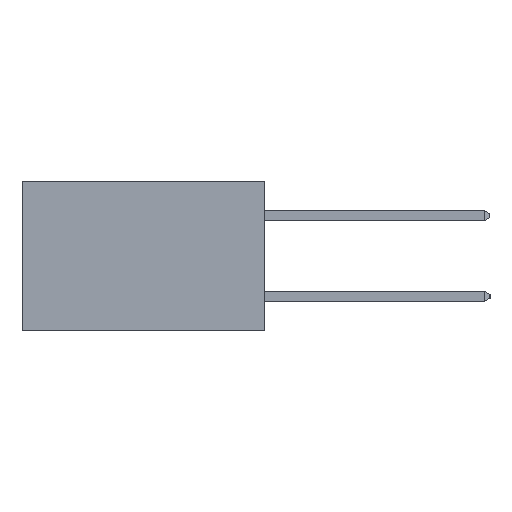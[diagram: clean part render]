
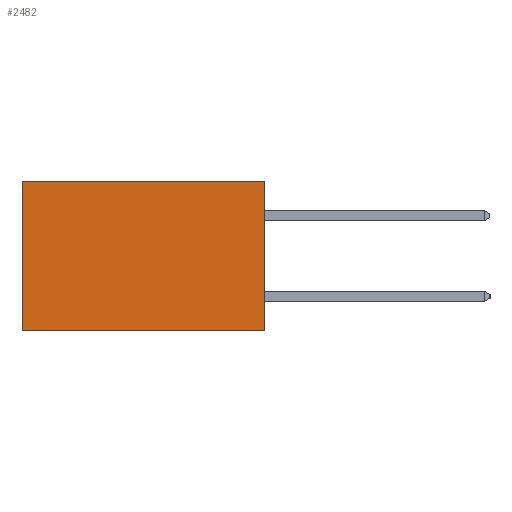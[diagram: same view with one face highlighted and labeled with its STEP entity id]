
A CAD part, left-side view. The second image highlights one B-rep face of the part: STEP entity #2482.
In plain terms, the highlighted planar face has unit normal (-1, 0, 0).
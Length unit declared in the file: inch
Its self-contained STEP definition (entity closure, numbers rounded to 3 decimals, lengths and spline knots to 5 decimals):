
#172 = ORIENTED_EDGE ( 'NONE', *, *, #15194, .T. ) ;
#1207 = DIRECTION ( 'NONE',  ( 0., 0., -1. ) ) ;
#1297 = DIRECTION ( 'NONE',  ( 1., 0., 0. ) ) ;
#1475 = CARTESIAN_POINT ( 'NONE',  ( 0.2615, 0., -0.37 ) ) ;
#1619 = PLANE ( 'NONE',  #10192 ) ;
#1718 = VECTOR ( 'NONE', #22442, 39.37008 ) ;
#2482 = ADVANCED_FACE ( 'NONE', ( #4401 ), #1619, .F. ) ;
#3646 = DIRECTION ( 'NONE',  ( 0., 1., 0. ) ) ;
#4401 = FACE_OUTER_BOUND ( 'NONE', #18795, .T. ) ;
#5141 = VERTEX_POINT ( 'NONE', #11143 ) ;
#7103 = VERTEX_POINT ( 'NONE', #10932 ) ;
#7178 = VECTOR ( 'NONE', #22992, 39.37008 ) ;
#7329 = EDGE_CURVE ( 'NONE', #7103, #5141, #19136, .T. ) ;
#7673 = VERTEX_POINT ( 'NONE', #11131 ) ;
#8150 = VECTOR ( 'NONE', #3646, 39.37008 ) ;
#8893 = ORIENTED_EDGE ( 'NONE', *, *, #15404, .T. ) ;
#10192 = AXIS2_PLACEMENT_3D ( 'NONE', #1475, #1297, #1207 ) ;
#10932 = CARTESIAN_POINT ( 'NONE',  ( 0.2615, 0., 0. ) ) ;
#11131 = CARTESIAN_POINT ( 'NONE',  ( 0.2615, 0.6, -0.37 ) ) ;
#11143 = CARTESIAN_POINT ( 'NONE',  ( 0.2615, 0., -0.37 ) ) ;
#12048 = LINE ( 'NONE', #20591, #1718 ) ;
#12344 = ORIENTED_EDGE ( 'NONE', *, *, #7329, .F. ) ;
#13279 = LINE ( 'NONE', #15151, #8150 ) ;
#13522 = VECTOR ( 'NONE', #20784, 39.37008 ) ;
#15151 = CARTESIAN_POINT ( 'NONE',  ( 0.2615, 0., -0.37 ) ) ;
#15194 = EDGE_CURVE ( 'NONE', #18160, #7673, #12048, .T. ) ;
#15404 = EDGE_CURVE ( 'NONE', #7103, #18160, #17366, .T. ) ;
#17070 = CARTESIAN_POINT ( 'NONE',  ( 0.2615, 0.6, 0. ) ) ;
#17366 = LINE ( 'NONE', #21149, #7178 ) ;
#18160 = VERTEX_POINT ( 'NONE', #17070 ) ;
#18795 = EDGE_LOOP ( 'NONE', ( #172, #22818, #12344, #8893 ) ) ;
#19136 = LINE ( 'NONE', #20917, #13522 ) ;
#20591 = CARTESIAN_POINT ( 'NONE',  ( 0.2615, 0.6, -0.37 ) ) ;
#20784 = DIRECTION ( 'NONE',  ( 0., 0., -1. ) ) ;
#20917 = CARTESIAN_POINT ( 'NONE',  ( 0.2615, 0., -0.37 ) ) ;
#21149 = CARTESIAN_POINT ( 'NONE',  ( 0.2615, 0., 0. ) ) ;
#21542 = EDGE_CURVE ( 'NONE', #5141, #7673, #13279, .T. ) ;
#22442 = DIRECTION ( 'NONE',  ( 0., 0., -1. ) ) ;
#22818 = ORIENTED_EDGE ( 'NONE', *, *, #21542, .F. ) ;
#22992 = DIRECTION ( 'NONE',  ( 0., 1., 0. ) ) ;
